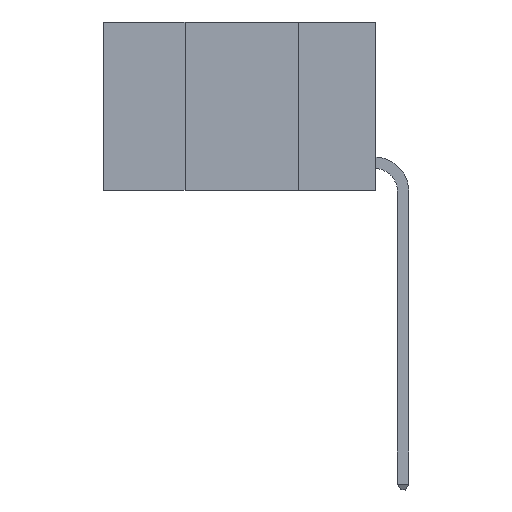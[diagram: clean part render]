
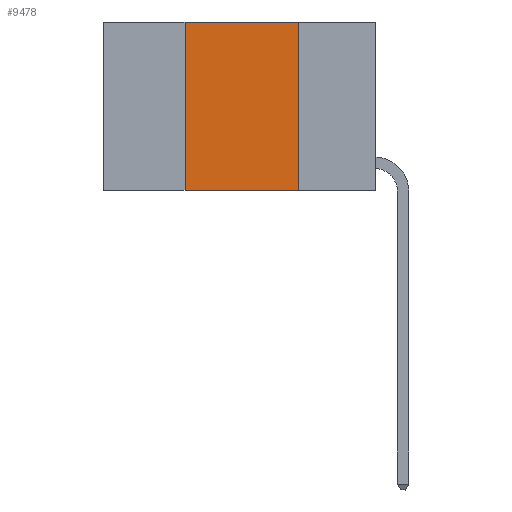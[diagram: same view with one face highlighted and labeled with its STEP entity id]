
A CAD part, left-side view. The second image highlights one B-rep face of the part: STEP entity #9478.
In plain terms, the highlighted planar face has unit normal (-1, 0, 0).
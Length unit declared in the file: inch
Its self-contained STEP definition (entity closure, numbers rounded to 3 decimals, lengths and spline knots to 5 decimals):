
#393 = DIRECTION ( 'NONE',  ( 0., -1., 0. ) ) ;
#510 = EDGE_CURVE ( 'NONE', #7206, #16548, #7755, .T. ) ;
#1074 = FACE_OUTER_BOUND ( 'NONE', #20468, .T. ) ;
#1117 = VECTOR ( 'NONE', #393, 39.37008 ) ;
#2316 = LINE ( 'NONE', #19816, #21088 ) ;
#5345 = DIRECTION ( 'NONE',  ( 0., 0., 1. ) ) ;
#6123 = LINE ( 'NONE', #22279, #15225 ) ;
#6230 = ORIENTED_EDGE ( 'NONE', *, *, #14453, .F. ) ;
#6404 = CARTESIAN_POINT ( 'NONE',  ( 0., 0.6, 0. ) ) ;
#7206 = VERTEX_POINT ( 'NONE', #11414 ) ;
#7755 = LINE ( 'NONE', #22189, #1117 ) ;
#7770 = CARTESIAN_POINT ( 'NONE',  ( 0., 0.17, -0.37 ) ) ;
#7902 = DIRECTION ( 'NONE',  ( 0., -1., 0. ) ) ;
#8265 = DIRECTION ( 'NONE',  ( 1., 0., 0. ) ) ;
#9376 = CARTESIAN_POINT ( 'NONE',  ( 0., 0.17, 0. ) ) ;
#9478 = ADVANCED_FACE ( 'NONE', ( #1074 ), #17292, .F. ) ;
#9809 = ORIENTED_EDGE ( 'NONE', *, *, #510, .F. ) ;
#10061 = AXIS2_PLACEMENT_3D ( 'NONE', #6404, #8265, #20889 ) ;
#11115 = EDGE_CURVE ( 'NONE', #16548, #18959, #11913, .T. ) ;
#11205 = DIRECTION ( 'NONE',  ( 0., 0., -1. ) ) ;
#11222 = VERTEX_POINT ( 'NONE', #16914 ) ;
#11414 = CARTESIAN_POINT ( 'NONE',  ( 0., 0.42, 0. ) ) ;
#11913 = LINE ( 'NONE', #9376, #16746 ) ;
#13224 = EDGE_CURVE ( 'NONE', #11222, #18959, #6123, .T. ) ;
#14453 = EDGE_CURVE ( 'NONE', #11222, #7206, #2316, .T. ) ;
#15225 = VECTOR ( 'NONE', #7902, 39.37008 ) ;
#16548 = VERTEX_POINT ( 'NONE', #20360 ) ;
#16746 = VECTOR ( 'NONE', #11205, 39.37008 ) ;
#16914 = CARTESIAN_POINT ( 'NONE',  ( 0., 0.42, -0.37 ) ) ;
#17292 = PLANE ( 'NONE',  #10061 ) ;
#18830 = ORIENTED_EDGE ( 'NONE', *, *, #11115, .F. ) ;
#18959 = VERTEX_POINT ( 'NONE', #7770 ) ;
#19577 = ORIENTED_EDGE ( 'NONE', *, *, #13224, .T. ) ;
#19816 = CARTESIAN_POINT ( 'NONE',  ( 0., 0.42, 0. ) ) ;
#20360 = CARTESIAN_POINT ( 'NONE',  ( 0., 0.17, 0. ) ) ;
#20468 = EDGE_LOOP ( 'NONE', ( #18830, #9809, #6230, #19577 ) ) ;
#20889 = DIRECTION ( 'NONE',  ( 0., 0., -1. ) ) ;
#21088 = VECTOR ( 'NONE', #5345, 39.37008 ) ;
#22189 = CARTESIAN_POINT ( 'NONE',  ( 0., 0.6, 0. ) ) ;
#22279 = CARTESIAN_POINT ( 'NONE',  ( 0., 0.6, -0.37 ) ) ;
